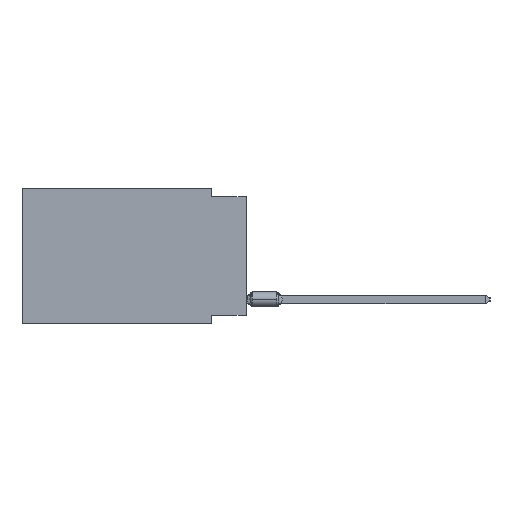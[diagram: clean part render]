
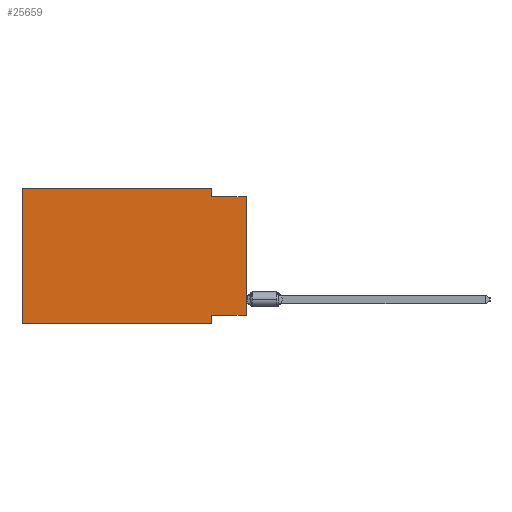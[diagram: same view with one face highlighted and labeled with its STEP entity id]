
A CAD part, left-side view. The second image highlights one B-rep face of the part: STEP entity #25659.
In plain terms, the highlighted planar face has unit normal (-1, 0, 0).
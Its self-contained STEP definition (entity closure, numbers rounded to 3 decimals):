
#75 = VERTEX_POINT ( 'NONE', #4798 ) ;
#394 = LINE ( 'NONE', #5654, #26449 ) ;
#486 = ORIENTED_EDGE ( 'NONE', *, *, #11910, .T. ) ;
#2090 = LINE ( 'NONE', #25770, #23053 ) ;
#2537 = CARTESIAN_POINT ( 'NONE',  ( 0., 2.54, -0.635 ) ) ;
#3029 = EDGE_CURVE ( 'NONE', #24294, #32870, #19251, .T. ) ;
#4558 = DIRECTION ( 'NONE',  ( 1., 0., 0. ) ) ;
#4798 = CARTESIAN_POINT ( 'NONE',  ( 0., 2.54, -9.271 ) ) ;
#4860 = VERTEX_POINT ( 'NONE', #20421 ) ;
#5389 = LINE ( 'NONE', #23832, #29173 ) ;
#5557 = VERTEX_POINT ( 'NONE', #18784 ) ;
#5654 = CARTESIAN_POINT ( 'NONE',  ( 0., 0., -0.635 ) ) ;
#5688 = EDGE_CURVE ( 'NONE', #5557, #75, #11389, .T. ) ;
#5761 = DIRECTION ( 'NONE',  ( 0., -1., 0. ) ) ;
#6651 = VECTOR ( 'NONE', #32822, 1000. ) ;
#6815 = LINE ( 'NONE', #17683, #31167 ) ;
#7176 = EDGE_LOOP ( 'NONE', ( #486, #28020, #16386, #34521, #9761, #15556, #22623, #28458 ) ) ;
#7742 = VECTOR ( 'NONE', #24194, 1000. ) ;
#9350 = EDGE_CURVE ( 'NONE', #17405, #24294, #26656, .T. ) ;
#9761 = ORIENTED_EDGE ( 'NONE', *, *, #9350, .F. ) ;
#9927 = VECTOR ( 'NONE', #5761, 1000. ) ;
#10166 = PLANE ( 'NONE',  #18014 ) ;
#11389 = LINE ( 'NONE', #22108, #6651 ) ;
#11888 = CARTESIAN_POINT ( 'NONE',  ( 0., 16.383, 0. ) ) ;
#11910 = EDGE_CURVE ( 'NONE', #5557, #13580, #5389, .T. ) ;
#12909 = EDGE_CURVE ( 'NONE', #75, #4860, #2090, .T. ) ;
#13580 = VERTEX_POINT ( 'NONE', #29817 ) ;
#15226 = LINE ( 'NONE', #28046, #30142 ) ;
#15256 = DIRECTION ( 'NONE',  ( 0., 0., -1. ) ) ;
#15556 = ORIENTED_EDGE ( 'NONE', *, *, #23599, .T. ) ;
#16352 = DIRECTION ( 'NONE',  ( 0., -1., 0. ) ) ;
#16386 = ORIENTED_EDGE ( 'NONE', *, *, #34664, .F. ) ;
#17179 = CARTESIAN_POINT ( 'NONE',  ( 0., 2.54, 0. ) ) ;
#17405 = VERTEX_POINT ( 'NONE', #33595 ) ;
#17683 = CARTESIAN_POINT ( 'NONE',  ( 0., 2.54, 0. ) ) ;
#18014 = AXIS2_PLACEMENT_3D ( 'NONE', #23682, #4558, #15256 ) ;
#18236 = CARTESIAN_POINT ( 'NONE',  ( 0., 16.383, 0. ) ) ;
#18784 = CARTESIAN_POINT ( 'NONE',  ( 0., 0., -9.271 ) ) ;
#19251 = LINE ( 'NONE', #11888, #9927 ) ;
#20421 = CARTESIAN_POINT ( 'NONE',  ( 0., 2.54, -9.906 ) ) ;
#20753 = EDGE_CURVE ( 'NONE', #33652, #13580, #394, .T. ) ;
#22108 = CARTESIAN_POINT ( 'NONE',  ( 0., 0., -9.271 ) ) ;
#22613 = DIRECTION ( 'NONE',  ( 0., -1., 0. ) ) ;
#22623 = ORIENTED_EDGE ( 'NONE', *, *, #12909, .F. ) ;
#23053 = VECTOR ( 'NONE', #34027, 1000. ) ;
#23599 = EDGE_CURVE ( 'NONE', #17405, #4860, #15226, .T. ) ;
#23682 = CARTESIAN_POINT ( 'NONE',  ( 0., 16.383, 0. ) ) ;
#23832 = CARTESIAN_POINT ( 'NONE',  ( 0., 0., 0. ) ) ;
#24194 = DIRECTION ( 'NONE',  ( 0., 0., 1. ) ) ;
#24294 = VERTEX_POINT ( 'NONE', #33366 ) ;
#25058 = DIRECTION ( 'NONE',  ( 0., 0., -1. ) ) ;
#25659 = ADVANCED_FACE ( 'NONE', ( #28591 ), #10166, .F. ) ;
#25770 = CARTESIAN_POINT ( 'NONE',  ( 0., 2.54, -9.906 ) ) ;
#26449 = VECTOR ( 'NONE', #16352, 1000. ) ;
#26656 = LINE ( 'NONE', #18236, #7742 ) ;
#28020 = ORIENTED_EDGE ( 'NONE', *, *, #20753, .F. ) ;
#28046 = CARTESIAN_POINT ( 'NONE',  ( 0., 16.383, -9.906 ) ) ;
#28458 = ORIENTED_EDGE ( 'NONE', *, *, #5688, .F. ) ;
#28591 = FACE_OUTER_BOUND ( 'NONE', #7176, .T. ) ;
#29173 = VECTOR ( 'NONE', #34544, 1000. ) ;
#29817 = CARTESIAN_POINT ( 'NONE',  ( 0., 0., -0.635 ) ) ;
#30142 = VECTOR ( 'NONE', #22613, 1000. ) ;
#31167 = VECTOR ( 'NONE', #25058, 1000. ) ;
#32822 = DIRECTION ( 'NONE',  ( 0., 1., 0. ) ) ;
#32870 = VERTEX_POINT ( 'NONE', #17179 ) ;
#33366 = CARTESIAN_POINT ( 'NONE',  ( 0., 16.383, 0. ) ) ;
#33595 = CARTESIAN_POINT ( 'NONE',  ( 0., 16.383, -9.906 ) ) ;
#33652 = VERTEX_POINT ( 'NONE', #2537 ) ;
#34027 = DIRECTION ( 'NONE',  ( 0., 0., -1. ) ) ;
#34521 = ORIENTED_EDGE ( 'NONE', *, *, #3029, .F. ) ;
#34544 = DIRECTION ( 'NONE',  ( 0., 0., 1. ) ) ;
#34664 = EDGE_CURVE ( 'NONE', #32870, #33652, #6815, .T. ) ;
